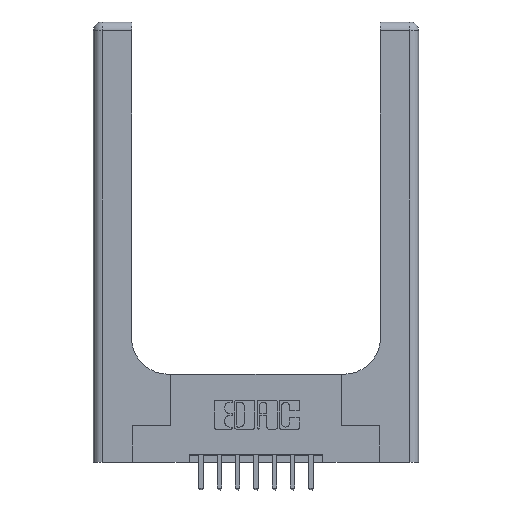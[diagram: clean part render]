
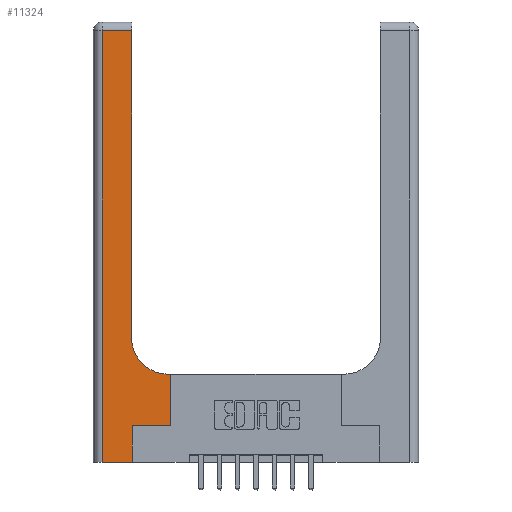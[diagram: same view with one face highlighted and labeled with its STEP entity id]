
A CAD part, top view. The second image highlights one B-rep face of the part: STEP entity #11324.
In plain terms, the highlighted planar face has unit normal (0, 0, 1).
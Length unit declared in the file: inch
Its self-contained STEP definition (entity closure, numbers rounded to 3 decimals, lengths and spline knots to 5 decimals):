
#245 = ORIENTED_EDGE ( 'NONE', *, *, #14640, .T. ) ;
#342 = FACE_OUTER_BOUND ( 'NONE', #8038, .T. ) ;
#407 = DIRECTION ( 'NONE',  ( 1., 0., 0. ) ) ;
#897 = EDGE_CURVE ( 'NONE', #4821, #2300, #13497, .T. ) ;
#1273 = ORIENTED_EDGE ( 'NONE', *, *, #2306, .T. ) ;
#1415 = DIRECTION ( 'NONE',  ( 0., 0., -1. ) ) ;
#1626 = LINE ( 'NONE', #3755, #14790 ) ;
#1756 = LINE ( 'NONE', #14599, #10634 ) ;
#1824 = CARTESIAN_POINT ( 'NONE',  ( 0.51, 0.6, 0.37 ) ) ;
#1944 = DIRECTION ( 'NONE',  ( -1., 0., 0. ) ) ;
#2244 = CARTESIAN_POINT ( 'NONE',  ( 0.06, 3., 0.37 ) ) ;
#2300 = VERTEX_POINT ( 'NONE', #12650 ) ;
#2306 = EDGE_CURVE ( 'NONE', #2300, #13123, #11659, .T. ) ;
#2373 = EDGE_CURVE ( 'NONE', #11274, #9429, #1626, .T. ) ;
#2549 = CIRCLE ( 'NONE', #2790, 0.25 ) ;
#2689 = EDGE_CURVE ( 'NONE', #9429, #3431, #10025, .T. ) ;
#2783 = EDGE_CURVE ( 'NONE', #12272, #4821, #11086, .T. ) ;
#2790 = AXIS2_PLACEMENT_3D ( 'NONE', #7563, #1415, #6053 ) ;
#2891 = DIRECTION ( 'NONE',  ( 1., 0., 0. ) ) ;
#3431 = VERTEX_POINT ( 'NONE', #7872 ) ;
#3755 = CARTESIAN_POINT ( 'NONE',  ( 0.265, 0.25, 0.37 ) ) ;
#3840 = PLANE ( 'NONE',  #4660 ) ;
#4331 = CARTESIAN_POINT ( 'NONE',  ( 0.26, 3., 0.37 ) ) ;
#4507 = VECTOR ( 'NONE', #14523, 39.37008 ) ;
#4660 = AXIS2_PLACEMENT_3D ( 'NONE', #14475, #9686, #14324 ) ;
#4821 = VERTEX_POINT ( 'NONE', #8843 ) ;
#4879 = ORIENTED_EDGE ( 'NONE', *, *, #2783, .T. ) ;
#5187 = LINE ( 'NONE', #13300, #4507 ) ;
#5274 = ORIENTED_EDGE ( 'NONE', *, *, #6789, .T. ) ;
#5329 = DIRECTION ( 'NONE',  ( 0., 1., 0. ) ) ;
#5969 = DIRECTION ( 'NONE',  ( 0., 1., 0. ) ) ;
#6053 = DIRECTION ( 'NONE',  ( 1., 0., 0. ) ) ;
#6193 = CARTESIAN_POINT ( 'NONE',  ( 0.265, 0.25, 0.37 ) ) ;
#6198 = CARTESIAN_POINT ( 'NONE',  ( 0.265, 0., 0.37 ) ) ;
#6427 = CARTESIAN_POINT ( 'NONE',  ( 0.26, 0.85, 0.37 ) ) ;
#6789 = EDGE_CURVE ( 'NONE', #14116, #11274, #13098, .T. ) ;
#6959 = DIRECTION ( 'NONE',  ( 0., -1., 0. ) ) ;
#7526 = CARTESIAN_POINT ( 'NONE',  ( 0.06, 0., 0.37 ) ) ;
#7563 = CARTESIAN_POINT ( 'NONE',  ( 0.51, 0.85, 0.37 ) ) ;
#7590 = CARTESIAN_POINT ( 'NONE',  ( 0.528, 0.25, 0.37 ) ) ;
#7723 = CARTESIAN_POINT ( 'NONE',  ( 0., 2.94, 0.37 ) ) ;
#7872 = CARTESIAN_POINT ( 'NONE',  ( 0.528, 0.6, 0.37 ) ) ;
#8023 = VECTOR ( 'NONE', #1944, 39.37008 ) ;
#8038 = EDGE_LOOP ( 'NONE', ( #4879, #11336, #1273, #8558, #5274, #13195, #10330, #245, #8042 ) ) ;
#8042 = ORIENTED_EDGE ( 'NONE', *, *, #14124, .T. ) ;
#8558 = ORIENTED_EDGE ( 'NONE', *, *, #9938, .T. ) ;
#8723 = DIRECTION ( 'NONE',  ( 0., 1., 0. ) ) ;
#8843 = CARTESIAN_POINT ( 'NONE',  ( 0.26, 2.94, 0.37 ) ) ;
#9429 = VERTEX_POINT ( 'NONE', #10831 ) ;
#9686 = DIRECTION ( 'NONE',  ( 0., 0., -1. ) ) ;
#9938 = EDGE_CURVE ( 'NONE', #13123, #14116, #1756, .T. ) ;
#10025 = LINE ( 'NONE', #7590, #12371 ) ;
#10299 = VECTOR ( 'NONE', #5969, 39.37008 ) ;
#10330 = ORIENTED_EDGE ( 'NONE', *, *, #2689, .T. ) ;
#10634 = VECTOR ( 'NONE', #2891, 39.37008 ) ;
#10831 = CARTESIAN_POINT ( 'NONE',  ( 0.528, 0.25, 0.37 ) ) ;
#11086 = LINE ( 'NONE', #4331, #11397 ) ;
#11274 = VERTEX_POINT ( 'NONE', #6193 ) ;
#11324 = ADVANCED_FACE ( 'NONE', ( #342 ), #3840, .F. ) ;
#11336 = ORIENTED_EDGE ( 'NONE', *, *, #897, .T. ) ;
#11397 = VECTOR ( 'NONE', #5329, 39.37008 ) ;
#11659 = LINE ( 'NONE', #2244, #14050 ) ;
#11962 = CARTESIAN_POINT ( 'NONE',  ( 0.265, 0., 0.37 ) ) ;
#12272 = VERTEX_POINT ( 'NONE', #6427 ) ;
#12371 = VECTOR ( 'NONE', #8723, 39.37008 ) ;
#12650 = CARTESIAN_POINT ( 'NONE',  ( 0.06, 2.94, 0.37 ) ) ;
#13098 = LINE ( 'NONE', #11962, #10299 ) ;
#13123 = VERTEX_POINT ( 'NONE', #7526 ) ;
#13195 = ORIENTED_EDGE ( 'NONE', *, *, #2373, .T. ) ;
#13300 = CARTESIAN_POINT ( 'NONE',  ( 0.26, 0.6, 0.37 ) ) ;
#13497 = LINE ( 'NONE', #7723, #8023 ) ;
#14050 = VECTOR ( 'NONE', #6959, 39.37008 ) ;
#14116 = VERTEX_POINT ( 'NONE', #6198 ) ;
#14124 = EDGE_CURVE ( 'NONE', #14519, #12272, #2549, .T. ) ;
#14324 = DIRECTION ( 'NONE',  ( -1., 0., 0. ) ) ;
#14475 = CARTESIAN_POINT ( 'NONE',  ( 0., 3., 0.37 ) ) ;
#14519 = VERTEX_POINT ( 'NONE', #1824 ) ;
#14523 = DIRECTION ( 'NONE',  ( -1., 0., 0. ) ) ;
#14599 = CARTESIAN_POINT ( 'NONE',  ( 0., 0., 0.37 ) ) ;
#14640 = EDGE_CURVE ( 'NONE', #3431, #14519, #5187, .T. ) ;
#14790 = VECTOR ( 'NONE', #407, 39.37008 ) ;
